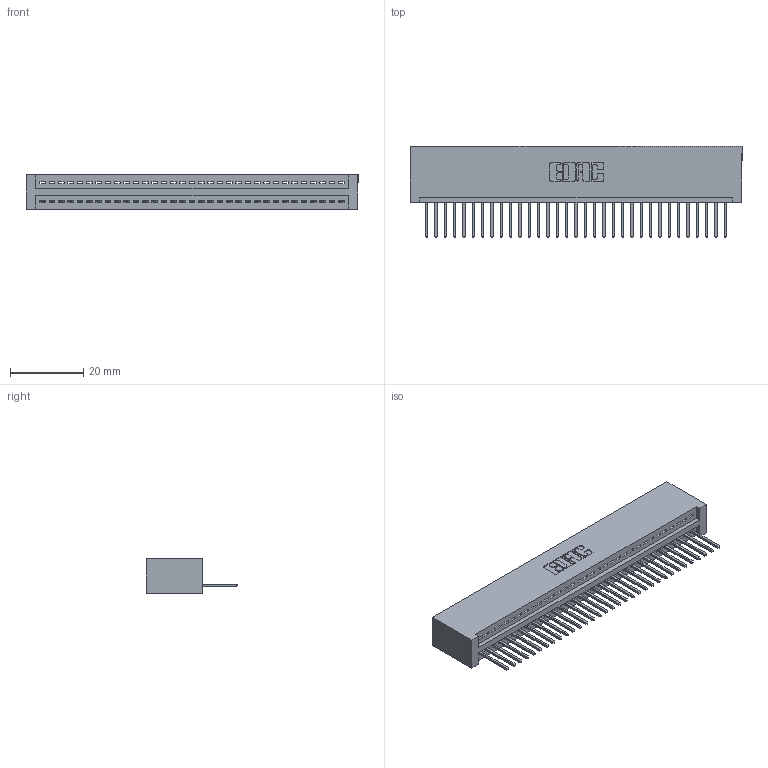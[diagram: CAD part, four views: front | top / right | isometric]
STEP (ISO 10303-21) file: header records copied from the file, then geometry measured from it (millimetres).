
FILE_DESCRIPTION (( 'STEP AP203' ), '1' );
FILE_NAME ('395-033-523-101.STEP', '2018-11-13T01:42:58', ( '' ), ( '' ), 'SwSTEP 2.0', 'SolidWorks 2016', '' );
FILE_SCHEMA (( 'CONFIG_CONTROL_DESIGN' ));
Length unit declared in the file: inch
Products named in the file (3): 345 Part_No Mounting Lugs; 345-292-001_345-293-123; 395-033-523-101
Assembly tree (34 placements, depth 2):
  395-033-523-101
    345 Part_No Mounting Lugs
    345-292-001_345-293-123  x33
Bounding box: 90.42 x 24.82 x 9.4 mm (x, y, z)
Volume: 9086.4 mm3; surface area: 12178.8 mm2
Topology: 34 solids, 34 shells, 2032 faces, 6125 edges, 4038 vertices
Faces by surface type: plane 1396, cylinder 636
Entity records: 25789 total; most frequent: CARTESIAN_POINT 4475, ORIENTED_EDGE 4442, DIRECTION 3915, EDGE_CURVE 2221, VECTOR 1965, LINE 1965, VERTEX_POINT 1478, AXIS2_PLACEMENT_3D 975
